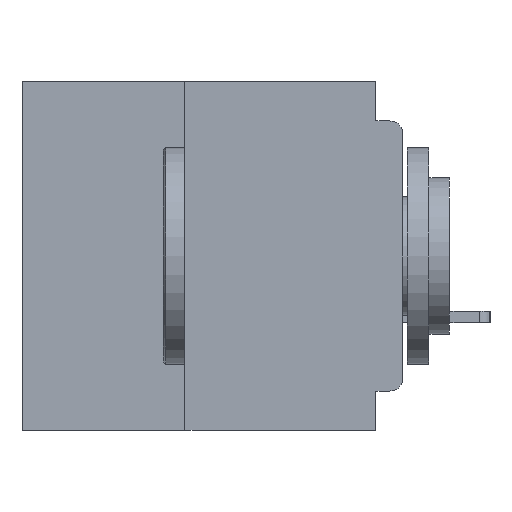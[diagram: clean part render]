
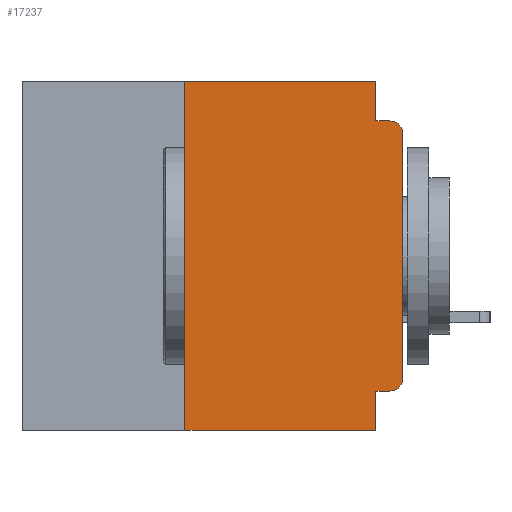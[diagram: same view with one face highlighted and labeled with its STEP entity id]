
A CAD part, left-side view. The second image highlights one B-rep face of the part: STEP entity #17237.
In plain terms, the highlighted planar face has unit normal (-1, 0, 0).
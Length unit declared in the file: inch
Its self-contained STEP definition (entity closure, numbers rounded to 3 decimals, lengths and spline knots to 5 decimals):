
#380 = DIRECTION ( 'NONE',  ( 0., 0., 1. ) ) ;
#601 = VERTEX_POINT ( 'NONE', #3421 ) ;
#1375 = CARTESIAN_POINT ( 'NONE',  ( 0., 0.031, -0.4 ) ) ;
#1528 = CARTESIAN_POINT ( 'NONE',  ( 0., 0.437, 0. ) ) ;
#1555 = EDGE_CURVE ( 'NONE', #8678, #30616, #6138, .T. ) ;
#2816 = ORIENTED_EDGE ( 'NONE', *, *, #25248, .F. ) ;
#2955 = AXIS2_PLACEMENT_3D ( 'NONE', #38747, #19061, #42045 ) ;
#3030 = DIRECTION ( 'NONE',  ( 0., 1., 0. ) ) ;
#3162 = VECTOR ( 'NONE', #3030, 39.37008 ) ;
#3421 = CARTESIAN_POINT ( 'NONE',  ( 0., 0.015, -0.355 ) ) ;
#3727 = ORIENTED_EDGE ( 'NONE', *, *, #30023, .T. ) ;
#4276 = VERTEX_POINT ( 'NONE', #12894 ) ;
#4312 = CARTESIAN_POINT ( 'NONE',  ( 0., 0.031, 0. ) ) ;
#4320 = VERTEX_POINT ( 'NONE', #16283 ) ;
#4983 = PLANE ( 'NONE',  #8631 ) ;
#6138 = LINE ( 'NONE', #22217, #31766 ) ;
#6427 = CARTESIAN_POINT ( 'NONE',  ( 0., 0., -0.355 ) ) ;
#6483 = CARTESIAN_POINT ( 'NONE',  ( 0., 0.015, -0.045 ) ) ;
#6757 = EDGE_CURVE ( 'NONE', #601, #11244, #29930, .T. ) ;
#6776 = VECTOR ( 'NONE', #36554, 39.37008 ) ;
#7549 = ORIENTED_EDGE ( 'NONE', *, *, #27975, .T. ) ;
#7832 = EDGE_CURVE ( 'NONE', #28512, #38246, #23712, .T. ) ;
#7835 = LINE ( 'NONE', #20019, #6776 ) ;
#8023 = VERTEX_POINT ( 'NONE', #17347 ) ;
#8408 = DIRECTION ( 'NONE',  ( 0., 0., -1. ) ) ;
#8631 = AXIS2_PLACEMENT_3D ( 'NONE', #1528, #15106, #8408 ) ;
#8678 = VERTEX_POINT ( 'NONE', #10493 ) ;
#8712 = CARTESIAN_POINT ( 'NONE',  ( 0., 0., -0.045 ) ) ;
#9089 = DIRECTION ( 'NONE',  ( -1., 0., 0. ) ) ;
#9224 = CARTESIAN_POINT ( 'NONE',  ( 0., 0.031, -0.355 ) ) ;
#9495 = CARTESIAN_POINT ( 'NONE',  ( 0., 0.437, -0.4 ) ) ;
#10493 = CARTESIAN_POINT ( 'NONE',  ( 0., 0.25, 0. ) ) ;
#11244 = VERTEX_POINT ( 'NONE', #9224 ) ;
#11339 = FACE_OUTER_BOUND ( 'NONE', #22395, .T. ) ;
#11527 = DIRECTION ( 'NONE',  ( 0., 0., -1. ) ) ;
#12211 = EDGE_CURVE ( 'NONE', #11244, #38246, #17921, .T. ) ;
#12554 = ORIENTED_EDGE ( 'NONE', *, *, #19707, .F. ) ;
#12659 = ORIENTED_EDGE ( 'NONE', *, *, #1555, .F. ) ;
#12894 = CARTESIAN_POINT ( 'NONE',  ( 0., 0., -0.34 ) ) ;
#13720 = VECTOR ( 'NONE', #26215, 39.37008 ) ;
#14890 = VECTOR ( 'NONE', #35335, 39.37008 ) ;
#15106 = DIRECTION ( 'NONE',  ( 1., 0., 0. ) ) ;
#15921 = LINE ( 'NONE', #8712, #14890 ) ;
#16064 = LINE ( 'NONE', #20726, #17142 ) ;
#16283 = CARTESIAN_POINT ( 'NONE',  ( 0., 0.031, -0.045 ) ) ;
#17023 = VERTEX_POINT ( 'NONE', #6483 ) ;
#17142 = VECTOR ( 'NONE', #380, 39.37008 ) ;
#17237 = ADVANCED_FACE ( 'NONE', ( #11339 ), #4983, .F. ) ;
#17347 = CARTESIAN_POINT ( 'NONE',  ( 0., 0., -0.06 ) ) ;
#17921 = LINE ( 'NONE', #1375, #18942 ) ;
#17932 = ORIENTED_EDGE ( 'NONE', *, *, #12211, .F. ) ;
#17960 = CIRCLE ( 'NONE', #2955, 0.015 ) ;
#17998 = EDGE_CURVE ( 'NONE', #601, #4276, #33114, .T. ) ;
#18396 = VECTOR ( 'NONE', #18632, 39.37008 ) ;
#18632 = DIRECTION ( 'NONE',  ( 0., 0., -1. ) ) ;
#18942 = VECTOR ( 'NONE', #11527, 39.37008 ) ;
#19061 = DIRECTION ( 'NONE',  ( -1., 0., 0. ) ) ;
#19707 = EDGE_CURVE ( 'NONE', #4320, #17023, #15921, .T. ) ;
#20019 = CARTESIAN_POINT ( 'NONE',  ( 0., 0.25, -0.4 ) ) ;
#20726 = CARTESIAN_POINT ( 'NONE',  ( 0., 0., 0. ) ) ;
#20989 = CARTESIAN_POINT ( 'NONE',  ( 0., 0.25, -0.4 ) ) ;
#21403 = ORIENTED_EDGE ( 'NONE', *, *, #6757, .F. ) ;
#21572 = EDGE_CURVE ( 'NONE', #30616, #4320, #28216, .T. ) ;
#22217 = CARTESIAN_POINT ( 'NONE',  ( 0., 0.437, 0. ) ) ;
#22395 = EDGE_LOOP ( 'NONE', ( #7549, #3727, #12554, #35956, #12659, #2816, #39957, #17932, #21403, #23019 ) ) ;
#22842 = DIRECTION ( 'NONE',  ( 0., -1., 0. ) ) ;
#23019 = ORIENTED_EDGE ( 'NONE', *, *, #17998, .T. ) ;
#23712 = LINE ( 'NONE', #9495, #13720 ) ;
#25248 = EDGE_CURVE ( 'NONE', #28512, #8678, #7835, .T. ) ;
#26215 = DIRECTION ( 'NONE',  ( 0., -1., 0. ) ) ;
#27975 = EDGE_CURVE ( 'NONE', #4276, #8023, #16064, .T. ) ;
#28216 = LINE ( 'NONE', #41628, #18396 ) ;
#28512 = VERTEX_POINT ( 'NONE', #20989 ) ;
#29105 = CARTESIAN_POINT ( 'NONE',  ( 0., 0.015, -0.34 ) ) ;
#29930 = LINE ( 'NONE', #6427, #3162 ) ;
#30023 = EDGE_CURVE ( 'NONE', #8023, #17023, #17960, .T. ) ;
#30616 = VERTEX_POINT ( 'NONE', #4312 ) ;
#31766 = VECTOR ( 'NONE', #22842, 39.37008 ) ;
#32414 = DIRECTION ( 'NONE',  ( 0., 0., -1. ) ) ;
#33114 = CIRCLE ( 'NONE', #33804, 0.015 ) ;
#33804 = AXIS2_PLACEMENT_3D ( 'NONE', #29105, #9089, #32414 ) ;
#34961 = CARTESIAN_POINT ( 'NONE',  ( 0., 0.031, -0.4 ) ) ;
#35335 = DIRECTION ( 'NONE',  ( 0., -1., 0. ) ) ;
#35956 = ORIENTED_EDGE ( 'NONE', *, *, #21572, .F. ) ;
#36554 = DIRECTION ( 'NONE',  ( 0., 0., 1. ) ) ;
#38246 = VERTEX_POINT ( 'NONE', #34961 ) ;
#38747 = CARTESIAN_POINT ( 'NONE',  ( 0., 0.015, -0.06 ) ) ;
#39957 = ORIENTED_EDGE ( 'NONE', *, *, #7832, .T. ) ;
#41628 = CARTESIAN_POINT ( 'NONE',  ( 0., 0.031, 0. ) ) ;
#42045 = DIRECTION ( 'NONE',  ( 0., 0., -1. ) ) ;
